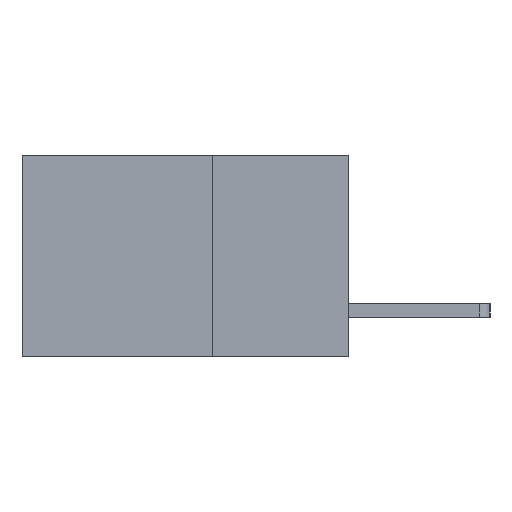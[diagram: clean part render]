
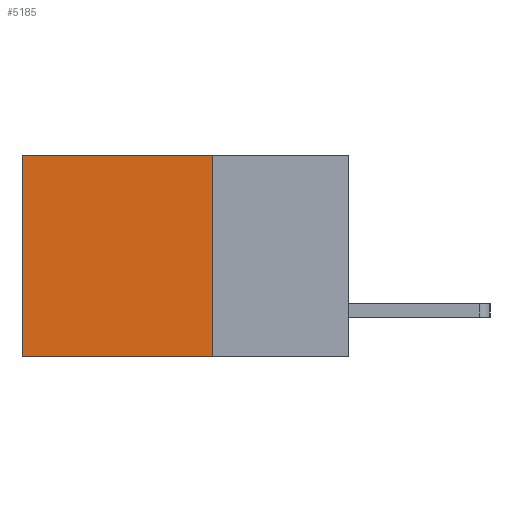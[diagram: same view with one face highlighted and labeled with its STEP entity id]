
A CAD part, left-side view. The second image highlights one B-rep face of the part: STEP entity #5185.
In plain terms, the highlighted planar face has unit normal (-1, 0, 0).
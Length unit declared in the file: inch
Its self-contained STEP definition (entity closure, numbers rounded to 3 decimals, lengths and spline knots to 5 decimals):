
#382 = VECTOR ( 'NONE', #4138, 39.37008 ) ;
#502 = DIRECTION ( 'NONE',  ( 1., 0., 0. ) ) ;
#541 = PLANE ( 'NONE',  #8160 ) ;
#545 = LINE ( 'NONE', #3059, #2793 ) ;
#2020 = CARTESIAN_POINT ( 'NONE',  ( 0.298, 0.6, 0. ) ) ;
#2100 = CARTESIAN_POINT ( 'NONE',  ( 0.298, 0.25, 0. ) ) ;
#2268 = EDGE_CURVE ( 'NONE', #3108, #2367, #7425, .T. ) ;
#2272 = FACE_OUTER_BOUND ( 'NONE', #9858, .T. ) ;
#2367 = VERTEX_POINT ( 'NONE', #2020 ) ;
#2634 = LINE ( 'NONE', #4764, #382 ) ;
#2793 = VECTOR ( 'NONE', #9744, 39.37008 ) ;
#3059 = CARTESIAN_POINT ( 'NONE',  ( 0.298, 0.25, 0. ) ) ;
#3108 = VERTEX_POINT ( 'NONE', #6133 ) ;
#3703 = CARTESIAN_POINT ( 'NONE',  ( 0.298, 0.6, -0.37 ) ) ;
#4071 = ORIENTED_EDGE ( 'NONE', *, *, #6584, .T. ) ;
#4138 = DIRECTION ( 'NONE',  ( 0., 0., -1. ) ) ;
#4223 = DIRECTION ( 'NONE',  ( 0., 1., 0. ) ) ;
#4764 = CARTESIAN_POINT ( 'NONE',  ( 0.298, 0.6, 0. ) ) ;
#5139 = EDGE_CURVE ( 'NONE', #3108, #8071, #545, .T. ) ;
#5185 = ADVANCED_FACE ( 'NONE', ( #2272 ), #541, .F. ) ;
#5374 = VECTOR ( 'NONE', #7107, 39.37008 ) ;
#5900 = ORIENTED_EDGE ( 'NONE', *, *, #7952, .F. ) ;
#6083 = CARTESIAN_POINT ( 'NONE',  ( 0.298, 0.25, 0. ) ) ;
#6133 = CARTESIAN_POINT ( 'NONE',  ( 0.298, 0.25, 0. ) ) ;
#6584 = EDGE_CURVE ( 'NONE', #2367, #6926, #2634, .T. ) ;
#6600 = CARTESIAN_POINT ( 'NONE',  ( 0.298, 0.25, -0.37 ) ) ;
#6926 = VERTEX_POINT ( 'NONE', #3703 ) ;
#7107 = DIRECTION ( 'NONE',  ( 0., 1., 0. ) ) ;
#7425 = LINE ( 'NONE', #6083, #5374 ) ;
#7657 = ORIENTED_EDGE ( 'NONE', *, *, #5139, .F. ) ;
#7831 = LINE ( 'NONE', #6600, #9573 ) ;
#7952 = EDGE_CURVE ( 'NONE', #8071, #6926, #7831, .T. ) ;
#8071 = VERTEX_POINT ( 'NONE', #9755 ) ;
#8160 = AXIS2_PLACEMENT_3D ( 'NONE', #2100, #502, #8596 ) ;
#8596 = DIRECTION ( 'NONE',  ( 0., 0., -1. ) ) ;
#9390 = ORIENTED_EDGE ( 'NONE', *, *, #2268, .T. ) ;
#9573 = VECTOR ( 'NONE', #4223, 39.37008 ) ;
#9744 = DIRECTION ( 'NONE',  ( 0., 0., -1. ) ) ;
#9755 = CARTESIAN_POINT ( 'NONE',  ( 0.298, 0.25, -0.37 ) ) ;
#9858 = EDGE_LOOP ( 'NONE', ( #4071, #5900, #7657, #9390 ) ) ;
